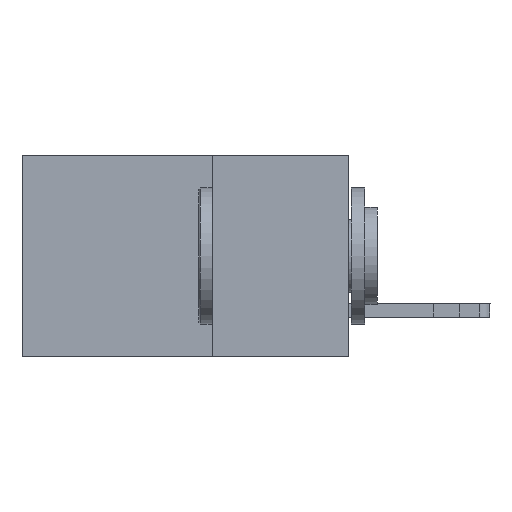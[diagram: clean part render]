
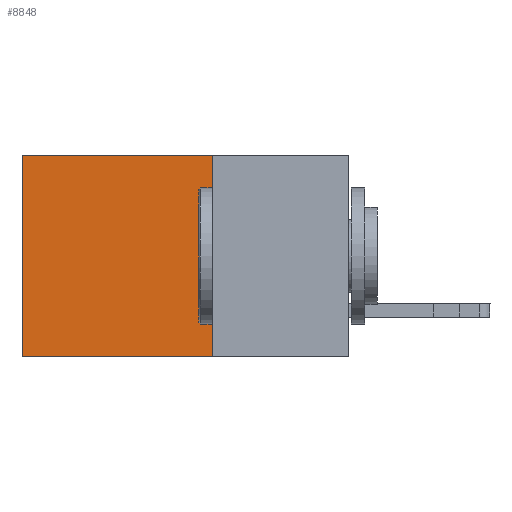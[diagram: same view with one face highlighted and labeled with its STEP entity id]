
A CAD part, left-side view. The second image highlights one B-rep face of the part: STEP entity #8848.
In plain terms, the highlighted planar face has unit normal (-1, 0, 0).
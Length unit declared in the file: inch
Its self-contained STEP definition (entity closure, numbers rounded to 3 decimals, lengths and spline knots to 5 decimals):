
#283 = AXIS2_PLACEMENT_3D ( 'NONE', #10364, #14150, #6621 ) ;
#371 = EDGE_CURVE ( 'NONE', #9891, #5191, #7599, .T. ) ;
#2190 = DIRECTION ( 'NONE',  ( 0., 0., -1. ) ) ;
#2244 = VECTOR ( 'NONE', #2190, 39.37008 ) ;
#2388 = VERTEX_POINT ( 'NONE', #9751 ) ;
#2776 = CARTESIAN_POINT ( 'NONE',  ( 0.2615, 0.25, 0. ) ) ;
#3386 = DIRECTION ( 'NONE',  ( 0., 1., 0. ) ) ;
#3733 = ORIENTED_EDGE ( 'NONE', *, *, #10814, .T. ) ;
#3846 = VECTOR ( 'NONE', #7242, 39.37008 ) ;
#4409 = LINE ( 'NONE', #2776, #10310 ) ;
#4475 = DIRECTION ( 'NONE',  ( 0., 0., -1. ) ) ;
#4545 = CARTESIAN_POINT ( 'NONE',  ( 0.2615, 0.25, -0.37 ) ) ;
#4908 = ORIENTED_EDGE ( 'NONE', *, *, #371, .F. ) ;
#5191 = VERTEX_POINT ( 'NONE', #14105 ) ;
#5372 = PLANE ( 'NONE',  #283 ) ;
#5558 = EDGE_CURVE ( 'NONE', #15026, #2388, #4409, .T. ) ;
#6584 = EDGE_CURVE ( 'NONE', #15026, #9891, #8724, .T. ) ;
#6621 = DIRECTION ( 'NONE',  ( 0., 0., -1. ) ) ;
#7242 = DIRECTION ( 'NONE',  ( 0., 1., 0. ) ) ;
#7478 = ORIENTED_EDGE ( 'NONE', *, *, #6584, .F. ) ;
#7599 = LINE ( 'NONE', #16139, #3846 ) ;
#8330 = VECTOR ( 'NONE', #4475, 39.37008 ) ;
#8475 = FACE_OUTER_BOUND ( 'NONE', #12378, .T. ) ;
#8724 = LINE ( 'NONE', #4545, #8330 ) ;
#8848 = ADVANCED_FACE ( 'NONE', ( #8475 ), #5372, .F. ) ;
#9751 = CARTESIAN_POINT ( 'NONE',  ( 0.2615, 0.6, 0. ) ) ;
#9891 = VERTEX_POINT ( 'NONE', #15144 ) ;
#10310 = VECTOR ( 'NONE', #3386, 39.37008 ) ;
#10364 = CARTESIAN_POINT ( 'NONE',  ( 0.2615, 0.25, -0.37 ) ) ;
#10814 = EDGE_CURVE ( 'NONE', #2388, #5191, #15204, .T. ) ;
#10994 = CARTESIAN_POINT ( 'NONE',  ( 0.2615, 0.6, -0.37 ) ) ;
#12378 = EDGE_LOOP ( 'NONE', ( #3733, #4908, #7478, #15533 ) ) ;
#13644 = CARTESIAN_POINT ( 'NONE',  ( 0.2615, 0.25, 0. ) ) ;
#14105 = CARTESIAN_POINT ( 'NONE',  ( 0.2615, 0.6, -0.37 ) ) ;
#14150 = DIRECTION ( 'NONE',  ( 1., 0., 0. ) ) ;
#15026 = VERTEX_POINT ( 'NONE', #13644 ) ;
#15144 = CARTESIAN_POINT ( 'NONE',  ( 0.2615, 0.25, -0.37 ) ) ;
#15204 = LINE ( 'NONE', #10994, #2244 ) ;
#15533 = ORIENTED_EDGE ( 'NONE', *, *, #5558, .T. ) ;
#16139 = CARTESIAN_POINT ( 'NONE',  ( 0.2615, 0.25, -0.37 ) ) ;
